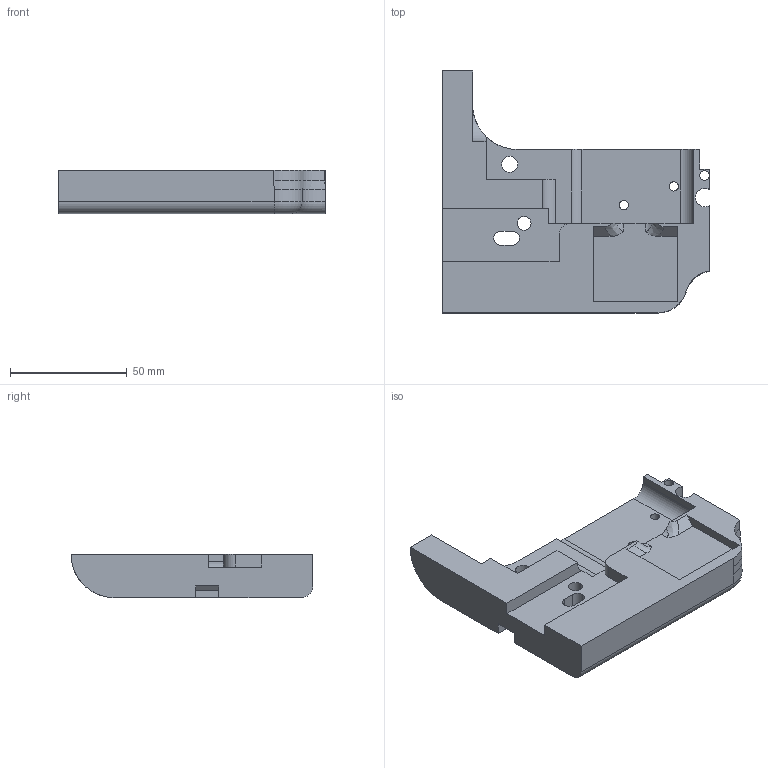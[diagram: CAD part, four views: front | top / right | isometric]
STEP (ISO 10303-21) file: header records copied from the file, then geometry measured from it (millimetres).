
FILE_DESCRIPTION (( 'STEP AP214' ), '1' );
FILE_NAME ('Receiver_FCG_Left.step', '2014-05-14T06:10:20', ( 'WarFairy' ), ( '' ), 'SwSTEP 2.0', 'SolidWorks 2013', '' );
FILE_SCHEMA (( 'AUTOMOTIVE_DESIGN' ));
Length unit declared in the file: inch
Products named in the file (1): Receiver_FCG_Left
Bounding box: 114.56 x 103.84 x 18.57 mm (x, y, z)
Volume: 116740.3 mm3; surface area: 27234.9 mm2
Topology: 1 solids, 1 shells, 111 faces, 308 edges, 200 vertices
Faces by surface type: plane 53, cylinder 48, torus 4, bspline 4, cone 1, sphere 1
Entity records: 3914 total; most frequent: CARTESIAN_POINT 985, ORIENTED_EDGE 614, DIRECTION 600, EDGE_CURVE 307, AXIS2_PLACEMENT_3D 207, VERTEX_POINT 200, LINE 186, VECTOR 186
